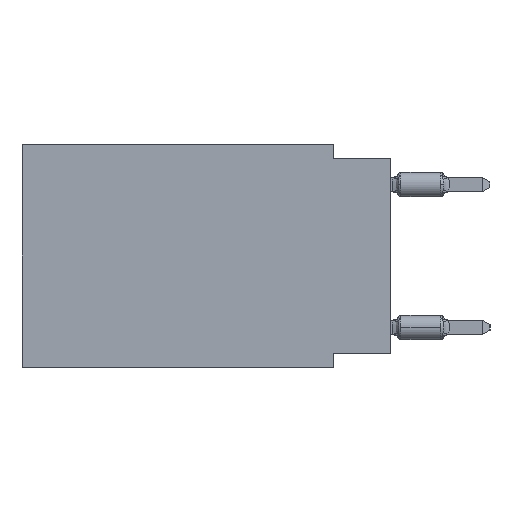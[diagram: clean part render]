
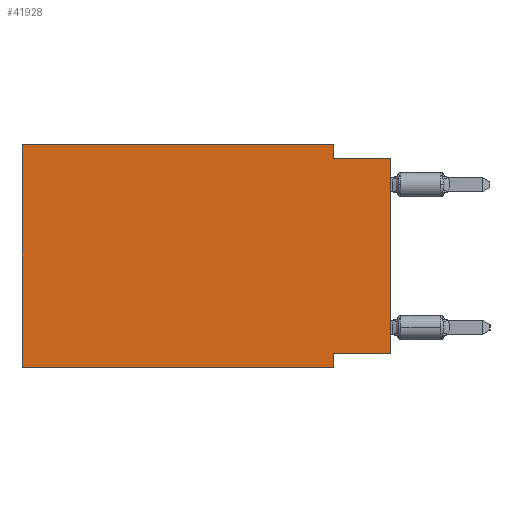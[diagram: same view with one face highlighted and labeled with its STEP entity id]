
A CAD part, left-side view. The second image highlights one B-rep face of the part: STEP entity #41928.
In plain terms, the highlighted planar face has unit normal (-1, 0, 0).
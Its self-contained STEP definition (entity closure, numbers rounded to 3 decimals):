
#578 = EDGE_CURVE ( 'NONE', #31391, #14085, #24185, .T. ) ;
#1964 = DIRECTION ( 'NONE',  ( 0., -1., 0. ) ) ;
#2139 = ORIENTED_EDGE ( 'NONE', *, *, #3406, .F. ) ;
#2734 = VECTOR ( 'NONE', #20075, 1000. ) ;
#3050 = CARTESIAN_POINT ( 'NONE',  ( 0., 2.54, 0. ) ) ;
#3262 = VERTEX_POINT ( 'NONE', #18145 ) ;
#3406 = EDGE_CURVE ( 'NONE', #3262, #26359, #43360, .T. ) ;
#4705 = PLANE ( 'NONE',  #4727 ) ;
#4727 = AXIS2_PLACEMENT_3D ( 'NONE', #12193, #25695, #32351 ) ;
#5087 = CARTESIAN_POINT ( 'NONE',  ( 0., 2.54, -9.271 ) ) ;
#5356 = ORIENTED_EDGE ( 'NONE', *, *, #29628, .F. ) ;
#7832 = ORIENTED_EDGE ( 'NONE', *, *, #9314, .F. ) ;
#9314 = EDGE_CURVE ( 'NONE', #26200, #33111, #43310, .T. ) ;
#9881 = LINE ( 'NONE', #10743, #21662 ) ;
#10743 = CARTESIAN_POINT ( 'NONE',  ( 0., 16.383, 0. ) ) ;
#11557 = FACE_OUTER_BOUND ( 'NONE', #40265, .T. ) ;
#12193 = CARTESIAN_POINT ( 'NONE',  ( 0., 16.383, 0. ) ) ;
#12767 = CARTESIAN_POINT ( 'NONE',  ( 0., 16.383, -9.906 ) ) ;
#12768 = LINE ( 'NONE', #20301, #2734 ) ;
#13218 = DIRECTION ( 'NONE',  ( 0., -1., 0. ) ) ;
#13695 = CARTESIAN_POINT ( 'NONE',  ( 0., 0., -9.271 ) ) ;
#14085 = VERTEX_POINT ( 'NONE', #14966 ) ;
#14349 = VECTOR ( 'NONE', #36077, 1000. ) ;
#14966 = CARTESIAN_POINT ( 'NONE',  ( 0., 16.383, 0. ) ) ;
#18145 = CARTESIAN_POINT ( 'NONE',  ( 0., 2.54, -0.635 ) ) ;
#18583 = ORIENTED_EDGE ( 'NONE', *, *, #32597, .F. ) ;
#20034 = VECTOR ( 'NONE', #13218, 1000. ) ;
#20075 = DIRECTION ( 'NONE',  ( 0., 0., -1. ) ) ;
#20144 = VECTOR ( 'NONE', #23147, 1000. ) ;
#20301 = CARTESIAN_POINT ( 'NONE',  ( 0., 2.54, -9.906 ) ) ;
#21543 = CARTESIAN_POINT ( 'NONE',  ( 0., 16.383, -9.906 ) ) ;
#21662 = VECTOR ( 'NONE', #23827, 1000. ) ;
#21910 = CARTESIAN_POINT ( 'NONE',  ( 0., 2.54, 0. ) ) ;
#23068 = VECTOR ( 'NONE', #32641, 1000. ) ;
#23147 = DIRECTION ( 'NONE',  ( 0., 1., 0. ) ) ;
#23827 = DIRECTION ( 'NONE',  ( 0., -1., 0. ) ) ;
#24045 = ORIENTED_EDGE ( 'NONE', *, *, #578, .F. ) ;
#24185 = LINE ( 'NONE', #37701, #25601 ) ;
#25601 = VECTOR ( 'NONE', #40607, 1000. ) ;
#25623 = CARTESIAN_POINT ( 'NONE',  ( 0., 0., -0.635 ) ) ;
#25695 = DIRECTION ( 'NONE',  ( 1., 0., 0. ) ) ;
#25798 = LINE ( 'NONE', #26226, #23068 ) ;
#26029 = VECTOR ( 'NONE', #1964, 1000. ) ;
#26200 = VERTEX_POINT ( 'NONE', #13695 ) ;
#26226 = CARTESIAN_POINT ( 'NONE',  ( 0., 0., 0. ) ) ;
#26359 = VERTEX_POINT ( 'NONE', #28936 ) ;
#27051 = ORIENTED_EDGE ( 'NONE', *, *, #27130, .F. ) ;
#27130 = EDGE_CURVE ( 'NONE', #36511, #3262, #32739, .T. ) ;
#27724 = EDGE_CURVE ( 'NONE', #31391, #34988, #29594, .T. ) ;
#28936 = CARTESIAN_POINT ( 'NONE',  ( 0., 0., -0.635 ) ) ;
#29111 = CARTESIAN_POINT ( 'NONE',  ( 0., 0., -9.271 ) ) ;
#29594 = LINE ( 'NONE', #12767, #20034 ) ;
#29628 = EDGE_CURVE ( 'NONE', #14085, #36511, #9881, .T. ) ;
#31391 = VERTEX_POINT ( 'NONE', #21543 ) ;
#32351 = DIRECTION ( 'NONE',  ( 0., 0., -1. ) ) ;
#32597 = EDGE_CURVE ( 'NONE', #33111, #34988, #12768, .T. ) ;
#32641 = DIRECTION ( 'NONE',  ( 0., 0., 1. ) ) ;
#32739 = LINE ( 'NONE', #21910, #14349 ) ;
#33111 = VERTEX_POINT ( 'NONE', #5087 ) ;
#34988 = VERTEX_POINT ( 'NONE', #37850 ) ;
#36077 = DIRECTION ( 'NONE',  ( 0., 0., -1. ) ) ;
#36511 = VERTEX_POINT ( 'NONE', #3050 ) ;
#37701 = CARTESIAN_POINT ( 'NONE',  ( 0., 16.383, 0. ) ) ;
#37850 = CARTESIAN_POINT ( 'NONE',  ( 0., 2.54, -9.906 ) ) ;
#38845 = ORIENTED_EDGE ( 'NONE', *, *, #27724, .T. ) ;
#40091 = EDGE_CURVE ( 'NONE', #26200, #26359, #25798, .T. ) ;
#40265 = EDGE_LOOP ( 'NONE', ( #43323, #2139, #27051, #5356, #24045, #38845, #18583, #7832 ) ) ;
#40607 = DIRECTION ( 'NONE',  ( 0., 0., 1. ) ) ;
#41928 = ADVANCED_FACE ( 'NONE', ( #11557 ), #4705, .F. ) ;
#43310 = LINE ( 'NONE', #29111, #20144 ) ;
#43323 = ORIENTED_EDGE ( 'NONE', *, *, #40091, .T. ) ;
#43360 = LINE ( 'NONE', #25623, #26029 ) ;
